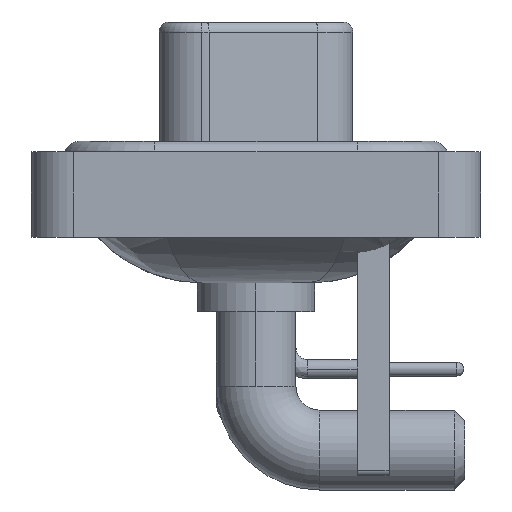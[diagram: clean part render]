
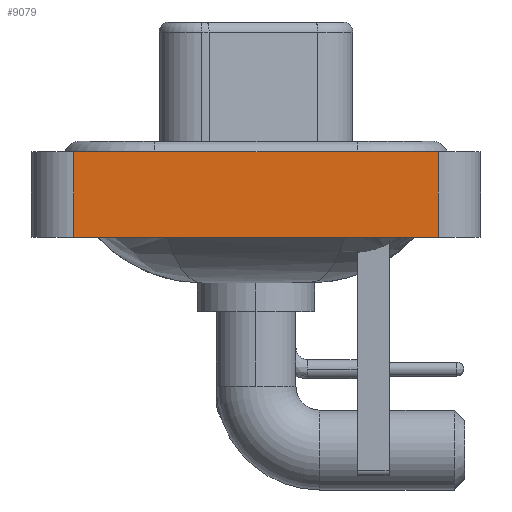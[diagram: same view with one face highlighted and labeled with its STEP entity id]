
A CAD part, left-side view. The second image highlights one B-rep face of the part: STEP entity #9079.
In plain terms, the highlighted planar face has unit normal (-1, 0, 0).
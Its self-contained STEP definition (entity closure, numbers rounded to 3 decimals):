
#286 = DIRECTION ( 'NONE',  ( 0., -1., 0. ) ) ;
#1135 = LINE ( 'NONE', #13884, #20545 ) ;
#1295 = CARTESIAN_POINT ( 'NONE',  ( -7.35, 8.55, -3.6 ) ) ;
#2337 = AXIS2_PLACEMENT_3D ( 'NONE', #19232, #27907, #8476 ) ;
#3941 = LINE ( 'NONE', #10449, #7815 ) ;
#4149 = EDGE_LOOP ( 'NONE', ( #25708, #19728, #26628, #25732 ) ) ;
#6677 = CARTESIAN_POINT ( 'NONE',  ( -7.35, -8.55, 0.4 ) ) ;
#7089 = EDGE_CURVE ( 'NONE', #10331, #20306, #1135, .T. ) ;
#7815 = VECTOR ( 'NONE', #12573, 1000. ) ;
#8476 = DIRECTION ( 'NONE',  ( 0., 0., 1. ) ) ;
#9079 = ADVANCED_FACE ( 'NONE', ( #24188 ), #13404, .T. ) ;
#9968 = EDGE_CURVE ( 'NONE', #22043, #20306, #22090, .T. ) ;
#10331 = VERTEX_POINT ( 'NONE', #10747 ) ;
#10449 = CARTESIAN_POINT ( 'NONE',  ( -7.35, -8.55, -3.6 ) ) ;
#10747 = CARTESIAN_POINT ( 'NONE',  ( -7.35, -8.55, -3.6 ) ) ;
#11185 = VECTOR ( 'NONE', #286, 1000. ) ;
#11765 = DIRECTION ( 'NONE',  ( 0., 0., 1. ) ) ;
#12468 = VERTEX_POINT ( 'NONE', #17297 ) ;
#12573 = DIRECTION ( 'NONE',  ( 0., -1., 0. ) ) ;
#13404 = PLANE ( 'NONE',  #2337 ) ;
#13884 = CARTESIAN_POINT ( 'NONE',  ( -7.35, -8.55, -3.6 ) ) ;
#14015 = CARTESIAN_POINT ( 'NONE',  ( -7.35, 8.55, 0.4 ) ) ;
#14043 = CARTESIAN_POINT ( 'NONE',  ( -7.35, -8.55, 0.4 ) ) ;
#16077 = EDGE_CURVE ( 'NONE', #12468, #10331, #3941, .T. ) ;
#17297 = CARTESIAN_POINT ( 'NONE',  ( -7.35, 8.55, -3.6 ) ) ;
#19002 = LINE ( 'NONE', #1295, #26721 ) ;
#19232 = CARTESIAN_POINT ( 'NONE',  ( -7.35, -8.55, -3.6 ) ) ;
#19728 = ORIENTED_EDGE ( 'NONE', *, *, #9968, .F. ) ;
#20306 = VERTEX_POINT ( 'NONE', #14043 ) ;
#20443 = EDGE_CURVE ( 'NONE', #12468, #22043, #19002, .T. ) ;
#20545 = VECTOR ( 'NONE', #11765, 1000. ) ;
#22043 = VERTEX_POINT ( 'NONE', #14015 ) ;
#22090 = LINE ( 'NONE', #6677, #11185 ) ;
#24188 = FACE_OUTER_BOUND ( 'NONE', #4149, .T. ) ;
#25708 = ORIENTED_EDGE ( 'NONE', *, *, #7089, .T. ) ;
#25732 = ORIENTED_EDGE ( 'NONE', *, *, #16077, .T. ) ;
#26628 = ORIENTED_EDGE ( 'NONE', *, *, #20443, .F. ) ;
#26721 = VECTOR ( 'NONE', #27686, 1000. ) ;
#27686 = DIRECTION ( 'NONE',  ( 0., 0., 1. ) ) ;
#27907 = DIRECTION ( 'NONE',  ( -1., 0., 0. ) ) ;
